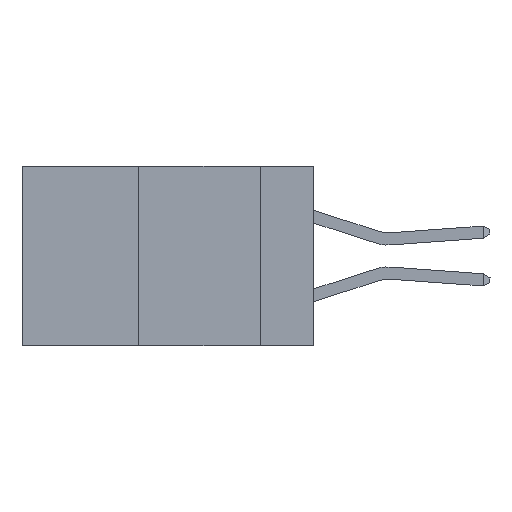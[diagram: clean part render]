
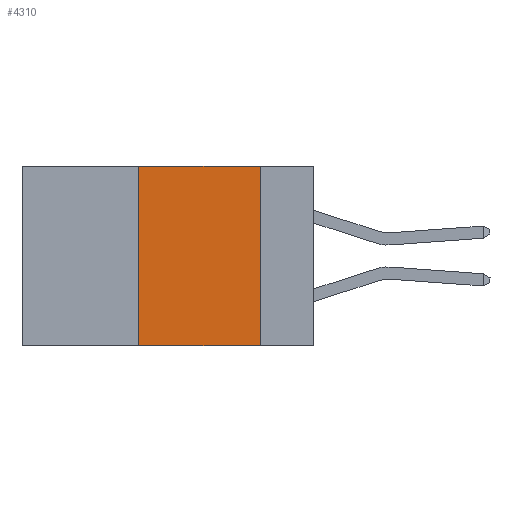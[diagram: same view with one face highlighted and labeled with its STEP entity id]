
A CAD part, left-side view. The second image highlights one B-rep face of the part: STEP entity #4310.
In plain terms, the highlighted planar face has unit normal (-1, 0, 0).
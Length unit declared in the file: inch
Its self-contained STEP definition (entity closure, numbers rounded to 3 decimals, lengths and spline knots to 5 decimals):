
#392 = DIRECTION ( 'NONE',  ( 0., 0., -1. ) ) ;
#478 = LINE ( 'NONE', #1691, #9293 ) ;
#815 = ORIENTED_EDGE ( 'NONE', *, *, #5877, .F. ) ;
#863 = LINE ( 'NONE', #7592, #5277 ) ;
#1360 = DIRECTION ( 'NONE',  ( 0., -1., 0. ) ) ;
#1401 = VECTOR ( 'NONE', #1360, 39.37008 ) ;
#1527 = DIRECTION ( 'NONE',  ( 0., 0., -1. ) ) ;
#1540 = DIRECTION ( 'NONE',  ( 1., 0., 0. ) ) ;
#1551 = ORIENTED_EDGE ( 'NONE', *, *, #7723, .F. ) ;
#1556 = PLANE ( 'NONE',  #3637 ) ;
#1652 = CARTESIAN_POINT ( 'NONE',  ( 0., 0.6, 0. ) ) ;
#1691 = CARTESIAN_POINT ( 'NONE',  ( 0., 0.6, -0.37 ) ) ;
#1827 = CARTESIAN_POINT ( 'NONE',  ( 0., 0.11, 0. ) ) ;
#1854 = VERTEX_POINT ( 'NONE', #1827 ) ;
#2241 = CARTESIAN_POINT ( 'NONE',  ( 0., 0.6, 0. ) ) ;
#2404 = ORIENTED_EDGE ( 'NONE', *, *, #9216, .F. ) ;
#2840 = ORIENTED_EDGE ( 'NONE', *, *, #8158, .T. ) ;
#2927 = CARTESIAN_POINT ( 'NONE',  ( 0., 0.36, 0. ) ) ;
#3472 = CARTESIAN_POINT ( 'NONE',  ( 0., 0.11, -0.37 ) ) ;
#3577 = LINE ( 'NONE', #3886, #7882 ) ;
#3637 = AXIS2_PLACEMENT_3D ( 'NONE', #1652, #1540, #1527 ) ;
#3886 = CARTESIAN_POINT ( 'NONE',  ( 0., 0.11, 0. ) ) ;
#4151 = VERTEX_POINT ( 'NONE', #2927 ) ;
#4174 = LINE ( 'NONE', #2241, #1401 ) ;
#4251 = EDGE_LOOP ( 'NONE', ( #815, #1551, #2404, #2840 ) ) ;
#4310 = ADVANCED_FACE ( 'NONE', ( #9612 ), #1556, .F. ) ;
#5277 = VECTOR ( 'NONE', #6760, 39.37008 ) ;
#5877 = EDGE_CURVE ( 'NONE', #1854, #6705, #3577, .T. ) ;
#6305 = VERTEX_POINT ( 'NONE', #8820 ) ;
#6705 = VERTEX_POINT ( 'NONE', #3472 ) ;
#6760 = DIRECTION ( 'NONE',  ( 0., 0., 1. ) ) ;
#7592 = CARTESIAN_POINT ( 'NONE',  ( 0., 0.36, 0. ) ) ;
#7723 = EDGE_CURVE ( 'NONE', #4151, #1854, #4174, .T. ) ;
#7882 = VECTOR ( 'NONE', #392, 39.37008 ) ;
#8158 = EDGE_CURVE ( 'NONE', #6305, #6705, #478, .T. ) ;
#8820 = CARTESIAN_POINT ( 'NONE',  ( 0., 0.36, -0.37 ) ) ;
#9216 = EDGE_CURVE ( 'NONE', #6305, #4151, #863, .T. ) ;
#9293 = VECTOR ( 'NONE', #10068, 39.37008 ) ;
#9612 = FACE_OUTER_BOUND ( 'NONE', #4251, .T. ) ;
#10068 = DIRECTION ( 'NONE',  ( 0., -1., 0. ) ) ;
